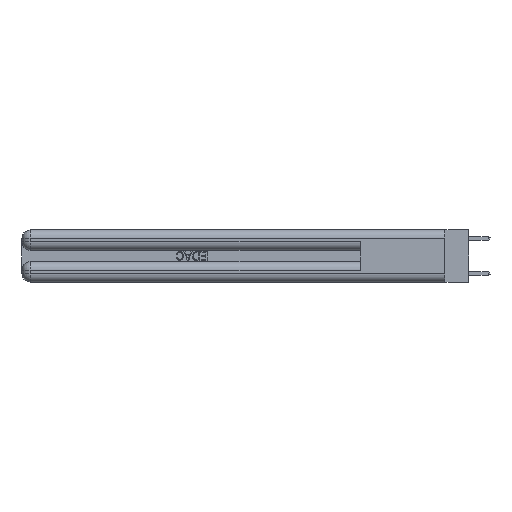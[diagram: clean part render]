
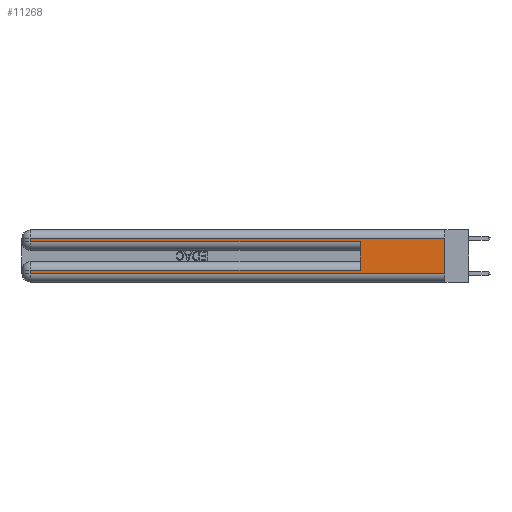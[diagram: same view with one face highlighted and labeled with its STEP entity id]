
A CAD part, left-side view. The second image highlights one B-rep face of the part: STEP entity #11268.
In plain terms, the highlighted planar face has unit normal (-1, 0, 0).
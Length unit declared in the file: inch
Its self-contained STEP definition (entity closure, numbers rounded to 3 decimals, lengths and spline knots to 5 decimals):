
#199 = CARTESIAN_POINT ( 'NONE',  ( 0., 0., 0.37 ) ) ;
#284 = LINE ( 'NONE', #3040, #30874 ) ;
#772 = EDGE_CURVE ( 'NONE', #31786, #7189, #23048, .T. ) ;
#1245 = LINE ( 'NONE', #12058, #25157 ) ;
#1731 = VERTEX_POINT ( 'NONE', #24371 ) ;
#1740 = CARTESIAN_POINT ( 'NONE',  ( 0., 2.94, 0.37 ) ) ;
#3040 = CARTESIAN_POINT ( 'NONE',  ( 0., 2.94, 0.37 ) ) ;
#3214 = VERTEX_POINT ( 'NONE', #7069 ) ;
#4789 = LINE ( 'NONE', #26680, #29688 ) ;
#5164 = DIRECTION ( 'NONE',  ( 0., 0., -1. ) ) ;
#5471 = ORIENTED_EDGE ( 'NONE', *, *, #30057, .T. ) ;
#5528 = PLANE ( 'NONE',  #10465 ) ;
#5656 = LINE ( 'NONE', #25359, #11881 ) ;
#5768 = VECTOR ( 'NONE', #6929, 39.37008 ) ;
#6141 = DIRECTION ( 'NONE',  ( 0., 0., -1. ) ) ;
#6929 = DIRECTION ( 'NONE',  ( 0., 0., 1. ) ) ;
#7069 = CARTESIAN_POINT ( 'NONE',  ( 0., 0.6, 0.285 ) ) ;
#7189 = VERTEX_POINT ( 'NONE', #30519 ) ;
#7861 = VECTOR ( 'NONE', #17689, 39.37008 ) ;
#7945 = CARTESIAN_POINT ( 'NONE',  ( 0., 2.94, 0.085 ) ) ;
#8449 = CARTESIAN_POINT ( 'NONE',  ( 0., 2.94, 0.06 ) ) ;
#8580 = DIRECTION ( 'NONE',  ( 0., 0., -1. ) ) ;
#9551 = VECTOR ( 'NONE', #8580, 39.37008 ) ;
#10143 = ORIENTED_EDGE ( 'NONE', *, *, #772, .T. ) ;
#10465 = AXIS2_PLACEMENT_3D ( 'NONE', #199, #13617, #5164 ) ;
#11268 = ADVANCED_FACE ( 'NONE', ( #16553 ), #5528, .F. ) ;
#11274 = VERTEX_POINT ( 'NONE', #8449 ) ;
#11550 = ORIENTED_EDGE ( 'NONE', *, *, #15496, .T. ) ;
#11881 = VECTOR ( 'NONE', #28628, 39.37008 ) ;
#12058 = CARTESIAN_POINT ( 'NONE',  ( 0., 0., 0.085 ) ) ;
#12304 = DIRECTION ( 'NONE',  ( 0., -1., 0. ) ) ;
#12561 = EDGE_CURVE ( 'NONE', #25243, #11274, #35200, .T. ) ;
#12858 = EDGE_LOOP ( 'NONE', ( #27102, #10143, #11550, #20156, #17059, #27309, #22771, #5471 ) ) ;
#13617 = DIRECTION ( 'NONE',  ( 1., 0., 0. ) ) ;
#15007 = DIRECTION ( 'NONE',  ( 0., 1., 0. ) ) ;
#15496 = EDGE_CURVE ( 'NONE', #7189, #1731, #284, .T. ) ;
#16553 = FACE_OUTER_BOUND ( 'NONE', #12858, .T. ) ;
#16841 = CARTESIAN_POINT ( 'NONE',  ( 0., 0.6, 0.085 ) ) ;
#17059 = ORIENTED_EDGE ( 'NONE', *, *, #34748, .F. ) ;
#17689 = DIRECTION ( 'NONE',  ( 0., 1., 0. ) ) ;
#19904 = VERTEX_POINT ( 'NONE', #16841 ) ;
#20156 = ORIENTED_EDGE ( 'NONE', *, *, #27459, .T. ) ;
#20372 = CARTESIAN_POINT ( 'NONE',  ( 0., 0., 0.31 ) ) ;
#22771 = ORIENTED_EDGE ( 'NONE', *, *, #12561, .T. ) ;
#23048 = LINE ( 'NONE', #34263, #7861 ) ;
#23619 = DIRECTION ( 'NONE',  ( 0., 0., -1. ) ) ;
#24151 = VERTEX_POINT ( 'NONE', #34238 ) ;
#24371 = CARTESIAN_POINT ( 'NONE',  ( 0., 2.94, 0.285 ) ) ;
#25157 = VECTOR ( 'NONE', #15007, 39.37008 ) ;
#25243 = VERTEX_POINT ( 'NONE', #7945 ) ;
#25359 = CARTESIAN_POINT ( 'NONE',  ( 0., 0., 0.285 ) ) ;
#26680 = CARTESIAN_POINT ( 'NONE',  ( 0., 0., 0.06 ) ) ;
#27102 = ORIENTED_EDGE ( 'NONE', *, *, #27342, .F. ) ;
#27309 = ORIENTED_EDGE ( 'NONE', *, *, #34722, .T. ) ;
#27342 = EDGE_CURVE ( 'NONE', #31786, #24151, #34165, .T. ) ;
#27459 = EDGE_CURVE ( 'NONE', #1731, #3214, #5656, .T. ) ;
#28446 = CARTESIAN_POINT ( 'NONE',  ( 0., 0., 0.37 ) ) ;
#28628 = DIRECTION ( 'NONE',  ( 0., -1., 0. ) ) ;
#29688 = VECTOR ( 'NONE', #12304, 39.37008 ) ;
#30057 = EDGE_CURVE ( 'NONE', #11274, #24151, #4789, .T. ) ;
#30519 = CARTESIAN_POINT ( 'NONE',  ( 0., 2.94, 0.31 ) ) ;
#30874 = VECTOR ( 'NONE', #6141, 39.37008 ) ;
#31786 = VERTEX_POINT ( 'NONE', #20372 ) ;
#32124 = LINE ( 'NONE', #34340, #5768 ) ;
#33429 = VECTOR ( 'NONE', #23619, 39.37008 ) ;
#34165 = LINE ( 'NONE', #28446, #9551 ) ;
#34238 = CARTESIAN_POINT ( 'NONE',  ( 0., 0., 0.06 ) ) ;
#34263 = CARTESIAN_POINT ( 'NONE',  ( 0., 0., 0.31 ) ) ;
#34340 = CARTESIAN_POINT ( 'NONE',  ( 0., 0.6, 0.145 ) ) ;
#34722 = EDGE_CURVE ( 'NONE', #19904, #25243, #1245, .T. ) ;
#34748 = EDGE_CURVE ( 'NONE', #19904, #3214, #32124, .T. ) ;
#35200 = LINE ( 'NONE', #1740, #33429 ) ;
